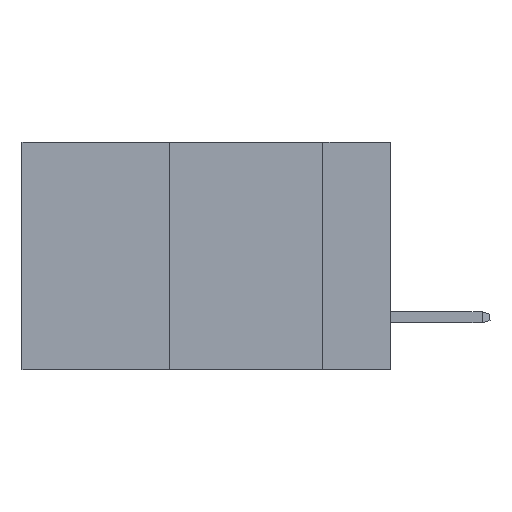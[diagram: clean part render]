
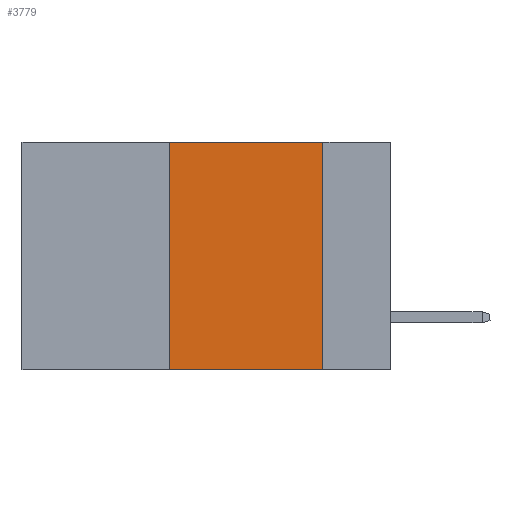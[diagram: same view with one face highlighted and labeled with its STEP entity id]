
A CAD part, left-side view. The second image highlights one B-rep face of the part: STEP entity #3779.
In plain terms, the highlighted planar face has unit normal (-1, 0, 0).
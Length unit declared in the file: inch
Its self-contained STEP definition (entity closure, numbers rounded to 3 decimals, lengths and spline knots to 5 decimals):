
#269 = DIRECTION ( 'NONE',  ( 0., -1., 0. ) ) ;
#848 = CARTESIAN_POINT ( 'NONE',  ( 0., 0.11, -0.37 ) ) ;
#2081 = VECTOR ( 'NONE', #269, 39.37008 ) ;
#2527 = AXIS2_PLACEMENT_3D ( 'NONE', #4155, #3474, #3354 ) ;
#2642 = LINE ( 'NONE', #10663, #10573 ) ;
#3307 = CARTESIAN_POINT ( 'NONE',  ( 0., 0.36, 0. ) ) ;
#3354 = DIRECTION ( 'NONE',  ( 0., 0., -1. ) ) ;
#3471 = LINE ( 'NONE', #5411, #8926 ) ;
#3474 = DIRECTION ( 'NONE',  ( 1., 0., 0. ) ) ;
#3779 = ADVANCED_FACE ( 'NONE', ( #13181 ), #3949, .F. ) ;
#3887 = VERTEX_POINT ( 'NONE', #848 ) ;
#3949 = PLANE ( 'NONE',  #2527 ) ;
#4155 = CARTESIAN_POINT ( 'NONE',  ( 0., 0.6, 0. ) ) ;
#4625 = VERTEX_POINT ( 'NONE', #12033 ) ;
#4824 = DIRECTION ( 'NONE',  ( 0., -1., 0. ) ) ;
#5052 = ORIENTED_EDGE ( 'NONE', *, *, #13842, .T. ) ;
#5384 = LINE ( 'NONE', #5991, #5767 ) ;
#5411 = CARTESIAN_POINT ( 'NONE',  ( 0., 0.6, 0. ) ) ;
#5767 = VECTOR ( 'NONE', #10068, 39.37008 ) ;
#5991 = CARTESIAN_POINT ( 'NONE',  ( 0., 0.11, 0. ) ) ;
#6147 = CARTESIAN_POINT ( 'NONE',  ( 0., 0.6, -0.37 ) ) ;
#6340 = EDGE_CURVE ( 'NONE', #13670, #4625, #3471, .T. ) ;
#7273 = ORIENTED_EDGE ( 'NONE', *, *, #13174, .F. ) ;
#7602 = ORIENTED_EDGE ( 'NONE', *, *, #6340, .F. ) ;
#8206 = EDGE_LOOP ( 'NONE', ( #7273, #7602, #10311, #5052 ) ) ;
#8926 = VECTOR ( 'NONE', #4824, 39.37008 ) ;
#10068 = DIRECTION ( 'NONE',  ( 0., 0., -1. ) ) ;
#10311 = ORIENTED_EDGE ( 'NONE', *, *, #13598, .F. ) ;
#10341 = VERTEX_POINT ( 'NONE', #12543 ) ;
#10573 = VECTOR ( 'NONE', #12616, 39.37008 ) ;
#10663 = CARTESIAN_POINT ( 'NONE',  ( 0., 0.36, 0. ) ) ;
#12033 = CARTESIAN_POINT ( 'NONE',  ( 0., 0.11, 0. ) ) ;
#12543 = CARTESIAN_POINT ( 'NONE',  ( 0., 0.36, -0.37 ) ) ;
#12616 = DIRECTION ( 'NONE',  ( 0., 0., 1. ) ) ;
#13174 = EDGE_CURVE ( 'NONE', #4625, #3887, #5384, .T. ) ;
#13181 = FACE_OUTER_BOUND ( 'NONE', #8206, .T. ) ;
#13294 = LINE ( 'NONE', #6147, #2081 ) ;
#13598 = EDGE_CURVE ( 'NONE', #10341, #13670, #2642, .T. ) ;
#13670 = VERTEX_POINT ( 'NONE', #3307 ) ;
#13842 = EDGE_CURVE ( 'NONE', #10341, #3887, #13294, .T. ) ;
